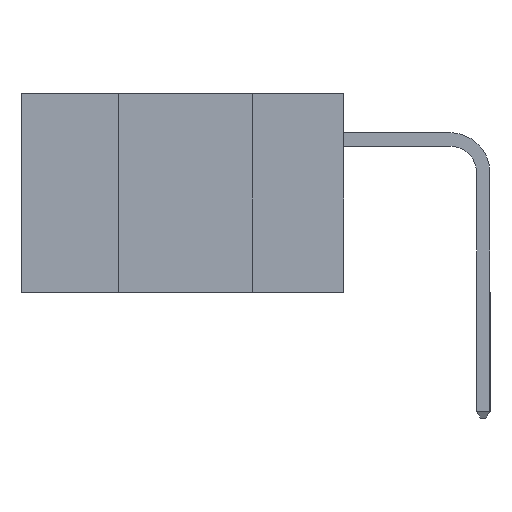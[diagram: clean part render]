
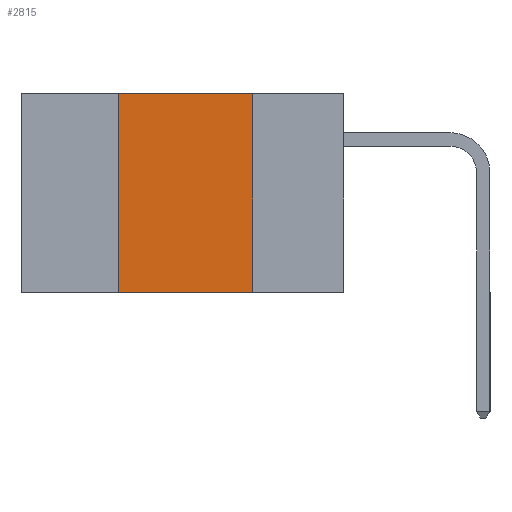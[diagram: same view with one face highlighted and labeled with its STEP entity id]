
A CAD part, left-side view. The second image highlights one B-rep face of the part: STEP entity #2815.
In plain terms, the highlighted planar face has unit normal (-1, 0, 0).
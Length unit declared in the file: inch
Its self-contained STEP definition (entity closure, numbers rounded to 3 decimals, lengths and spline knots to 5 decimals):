
#693 = VECTOR ( 'NONE', #1806, 39.37008 ) ;
#1091 = DIRECTION ( 'NONE',  ( 0., -1., 0. ) ) ;
#1771 = LINE ( 'NONE', #18280, #14754 ) ;
#1806 = DIRECTION ( 'NONE',  ( 0., -1., 0. ) ) ;
#2815 = ADVANCED_FACE ( 'NONE', ( #12211 ), #11394, .F. ) ;
#3166 = VECTOR ( 'NONE', #14970, 39.37008 ) ;
#3221 = VECTOR ( 'NONE', #1091, 39.37008 ) ;
#3392 = ORIENTED_EDGE ( 'NONE', *, *, #12504, .F. ) ;
#3602 = LINE ( 'NONE', #13666, #693 ) ;
#4918 = ORIENTED_EDGE ( 'NONE', *, *, #10924, .F. ) ;
#5678 = ORIENTED_EDGE ( 'NONE', *, *, #18077, .F. ) ;
#6381 = CARTESIAN_POINT ( 'NONE',  ( 0., 0.42, 0. ) ) ;
#6470 = DIRECTION ( 'NONE',  ( 0., 0., -1. ) ) ;
#8177 = LINE ( 'NONE', #6381, #3166 ) ;
#8625 = CARTESIAN_POINT ( 'NONE',  ( 0., 0.42, -0.37 ) ) ;
#10436 = VERTEX_POINT ( 'NONE', #12051 ) ;
#10440 = AXIS2_PLACEMENT_3D ( 'NONE', #11373, #11233, #11083 ) ;
#10924 = EDGE_CURVE ( 'NONE', #13335, #13527, #8177, .T. ) ;
#11083 = DIRECTION ( 'NONE',  ( 0., 0., -1. ) ) ;
#11233 = DIRECTION ( 'NONE',  ( 1., 0., 0. ) ) ;
#11373 = CARTESIAN_POINT ( 'NONE',  ( 0., 0.6, 0. ) ) ;
#11394 = PLANE ( 'NONE',  #10440 ) ;
#11499 = CARTESIAN_POINT ( 'NONE',  ( 0., 0.17, -0.37 ) ) ;
#12051 = CARTESIAN_POINT ( 'NONE',  ( 0., 0.17, 0. ) ) ;
#12211 = FACE_OUTER_BOUND ( 'NONE', #14997, .T. ) ;
#12504 = EDGE_CURVE ( 'NONE', #10436, #15163, #1771, .T. ) ;
#12650 = EDGE_CURVE ( 'NONE', #13335, #15163, #3602, .T. ) ;
#13335 = VERTEX_POINT ( 'NONE', #8625 ) ;
#13527 = VERTEX_POINT ( 'NONE', #19257 ) ;
#13666 = CARTESIAN_POINT ( 'NONE',  ( 0., 0.6, -0.37 ) ) ;
#14754 = VECTOR ( 'NONE', #6470, 39.37008 ) ;
#14970 = DIRECTION ( 'NONE',  ( 0., 0., 1. ) ) ;
#14997 = EDGE_LOOP ( 'NONE', ( #3392, #5678, #4918, #19825 ) ) ;
#15163 = VERTEX_POINT ( 'NONE', #11499 ) ;
#16263 = CARTESIAN_POINT ( 'NONE',  ( 0., 0.6, 0. ) ) ;
#18077 = EDGE_CURVE ( 'NONE', #13527, #10436, #20933, .T. ) ;
#18280 = CARTESIAN_POINT ( 'NONE',  ( 0., 0.17, 0. ) ) ;
#19257 = CARTESIAN_POINT ( 'NONE',  ( 0., 0.42, 0. ) ) ;
#19825 = ORIENTED_EDGE ( 'NONE', *, *, #12650, .T. ) ;
#20933 = LINE ( 'NONE', #16263, #3221 ) ;
